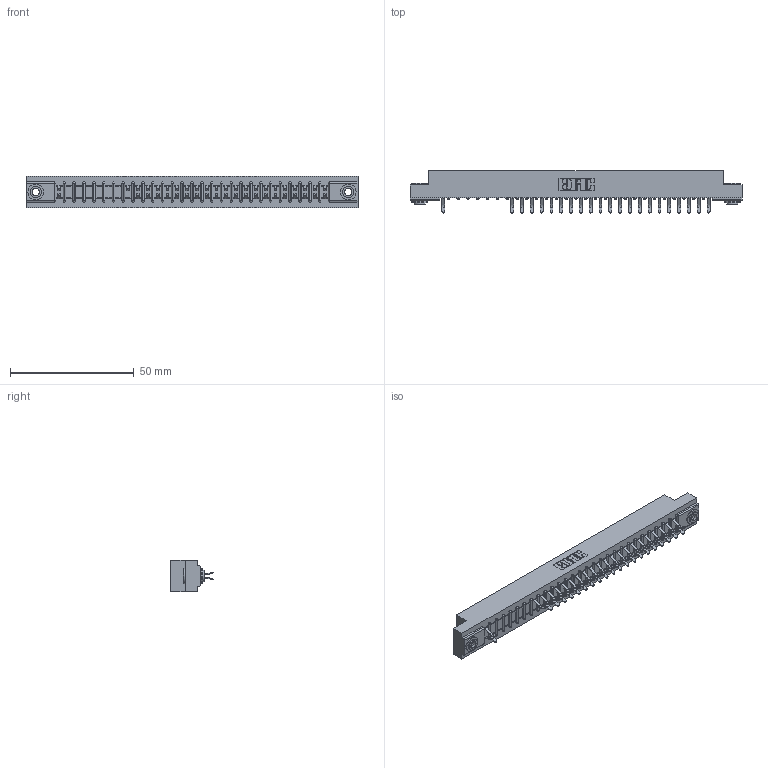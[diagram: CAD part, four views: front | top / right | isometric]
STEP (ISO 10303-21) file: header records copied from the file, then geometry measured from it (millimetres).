
FILE_DESCRIPTION (( 'STEP AP203' ), '1' );
FILE_NAME ('307-056-556-203.STEP', '2018-08-06T07:00:14', ( '' ), ( '' ), 'SwSTEP 2.0', 'SolidWorks 2016', '' );
FILE_SCHEMA (( 'CONFIG_CONTROL_DESIGN' ));
Length unit declared in the file: inch
Products named in the file (4): 307-290-001_556; 345-250-002_345-250-002-102; 307-056-556-203; 307 Part_.156 Dia Mounting Holes
Assembly tree (46 placements, depth 2):
  307-056-556-203
    307 Part_.156 Dia Mounting Holes
    307-290-001_556  x43
    345-250-002_345-250-002-102  x2
Bounding box: 133.96 x 16.97 x 12.7 mm (x, y, z)
Volume: 13971 mm3; surface area: 15843.7 mm2
Topology: 46 solids, 46 shells, 2479 faces, 6957 edges, 4498 vertices
Faces by surface type: plane 1591, cylinder 822, sphere 58, cone 8
Entity records: 27379 total; most frequent: CARTESIAN_POINT 4520, ORIENTED_EDGE 4482, DIRECTION 4435, EDGE_CURVE 2241, LINE 1705, VECTOR 1705, VERTEX_POINT 1450, AXIS2_PLACEMENT_3D 1365
